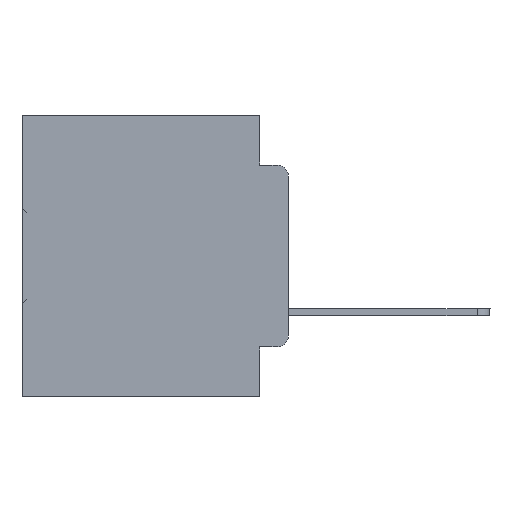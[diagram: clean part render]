
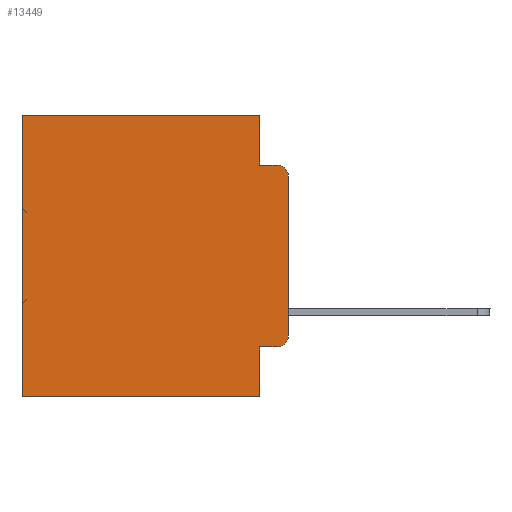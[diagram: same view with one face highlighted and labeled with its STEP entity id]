
A CAD part, left-side view. The second image highlights one B-rep face of the part: STEP entity #13449.
In plain terms, the highlighted planar face has unit normal (-1, 0, 0).
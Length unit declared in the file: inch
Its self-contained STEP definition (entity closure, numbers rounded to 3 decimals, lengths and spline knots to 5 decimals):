
#15 = CARTESIAN_POINT ( 'NONE',  ( 0.298, 0.051, -0.4115 ) ) ;
#1061 = ORIENTED_EDGE ( 'NONE', *, *, #3541, .F. ) ;
#1403 = FACE_OUTER_BOUND ( 'NONE', #36250, .T. ) ;
#1502 = CARTESIAN_POINT ( 'NONE',  ( 0.298, 0.051, -0.0885 ) ) ;
#1765 = AXIS2_PLACEMENT_3D ( 'NONE', #23868, #29611, #15576 ) ;
#1798 = LINE ( 'NONE', #21835, #19086 ) ;
#1844 = EDGE_CURVE ( 'NONE', #3510, #11392, #1798, .T. ) ;
#2751 = VECTOR ( 'NONE', #7389, 39.37008 ) ;
#3070 = CARTESIAN_POINT ( 'NONE',  ( 0.298, 0.473, -0.5 ) ) ;
#3287 = CARTESIAN_POINT ( 'NONE',  ( 0.298, 0., -0.1085 ) ) ;
#3510 = VERTEX_POINT ( 'NONE', #24153 ) ;
#3541 = EDGE_CURVE ( 'NONE', #10267, #5539, #7204, .T. ) ;
#3758 = CARTESIAN_POINT ( 'NONE',  ( 0.298, 0.02, -0.0885 ) ) ;
#4334 = VERTEX_POINT ( 'NONE', #31957 ) ;
#5153 = EDGE_CURVE ( 'NONE', #26758, #6152, #29954, .T. ) ;
#5460 = DIRECTION ( 'NONE',  ( -1., 0., 0. ) ) ;
#5539 = VERTEX_POINT ( 'NONE', #3070 ) ;
#5922 = EDGE_CURVE ( 'NONE', #33526, #5539, #17588, .T. ) ;
#6152 = VERTEX_POINT ( 'NONE', #3758 ) ;
#6642 = LINE ( 'NONE', #1502, #9301 ) ;
#7204 = LINE ( 'NONE', #13098, #2751 ) ;
#7389 = DIRECTION ( 'NONE',  ( 0., 1., 0. ) ) ;
#7728 = CARTESIAN_POINT ( 'NONE',  ( 0.298, 0.051, 0. ) ) ;
#8185 = DIRECTION ( 'NONE',  ( 0., 0., -1. ) ) ;
#8460 = EDGE_CURVE ( 'NONE', #3510, #33526, #17538, .T. ) ;
#8708 = VECTOR ( 'NONE', #18972, 39.37008 ) ;
#8750 = CARTESIAN_POINT ( 'NONE',  ( 0.298, 0.02, -0.3915 ) ) ;
#9301 = VECTOR ( 'NONE', #35219, 39.37008 ) ;
#9411 = CARTESIAN_POINT ( 'NONE',  ( 0.298, 0., 0. ) ) ;
#10267 = VERTEX_POINT ( 'NONE', #18409 ) ;
#10815 = DIRECTION ( 'NONE',  ( 0., 0., -1. ) ) ;
#11392 = VERTEX_POINT ( 'NONE', #24156 ) ;
#11633 = ORIENTED_EDGE ( 'NONE', *, *, #12539, .F. ) ;
#11670 = CARTESIAN_POINT ( 'NONE',  ( 0.298, 0.051, -0.4115 ) ) ;
#12088 = ORIENTED_EDGE ( 'NONE', *, *, #12703, .F. ) ;
#12374 = VECTOR ( 'NONE', #25185, 39.37008 ) ;
#12539 = EDGE_CURVE ( 'NONE', #11392, #6152, #6642, .T. ) ;
#12648 = PLANE ( 'NONE',  #1765 ) ;
#12703 = EDGE_CURVE ( 'NONE', #13671, #10267, #13623, .T. ) ;
#13098 = CARTESIAN_POINT ( 'NONE',  ( 0.298, 0., -0.5 ) ) ;
#13236 = CARTESIAN_POINT ( 'NONE',  ( 0.298, 0., 0. ) ) ;
#13449 = ADVANCED_FACE ( 'NONE', ( #1403 ), #12648, .F. ) ;
#13495 = ORIENTED_EDGE ( 'NONE', *, *, #1844, .F. ) ;
#13623 = LINE ( 'NONE', #7728, #8708 ) ;
#13671 = VERTEX_POINT ( 'NONE', #11670 ) ;
#14022 = ORIENTED_EDGE ( 'NONE', *, *, #8460, .T. ) ;
#14121 = ORIENTED_EDGE ( 'NONE', *, *, #5922, .T. ) ;
#14278 = ORIENTED_EDGE ( 'NONE', *, *, #5153, .T. ) ;
#14392 = EDGE_CURVE ( 'NONE', #26758, #17252, #27607, .T. ) ;
#14890 = CARTESIAN_POINT ( 'NONE',  ( 0.298, 0.02, -0.1085 ) ) ;
#15576 = DIRECTION ( 'NONE',  ( 0., 0., -1. ) ) ;
#16735 = ORIENTED_EDGE ( 'NONE', *, *, #14392, .F. ) ;
#16777 = LINE ( 'NONE', #15, #19523 ) ;
#16954 = DIRECTION ( 'NONE',  ( 0., -1., 0. ) ) ;
#17252 = VERTEX_POINT ( 'NONE', #24228 ) ;
#17538 = LINE ( 'NONE', #9411, #27428 ) ;
#17588 = LINE ( 'NONE', #20335, #26091 ) ;
#18409 = CARTESIAN_POINT ( 'NONE',  ( 0.298, 0.051, -0.5 ) ) ;
#18936 = EDGE_CURVE ( 'NONE', #4334, #17252, #34670, .T. ) ;
#18972 = DIRECTION ( 'NONE',  ( 0., 0., -1. ) ) ;
#19086 = VECTOR ( 'NONE', #8185, 39.37008 ) ;
#19523 = VECTOR ( 'NONE', #16954, 39.37008 ) ;
#20335 = CARTESIAN_POINT ( 'NONE',  ( 0.298, 0.473, 0. ) ) ;
#21713 = EDGE_CURVE ( 'NONE', #13671, #4334, #16777, .T. ) ;
#21835 = CARTESIAN_POINT ( 'NONE',  ( 0.298, 0.051, 0. ) ) ;
#22532 = DIRECTION ( 'NONE',  ( 0., 0., -1. ) ) ;
#23868 = CARTESIAN_POINT ( 'NONE',  ( 0.298, 0., 0. ) ) ;
#24037 = AXIS2_PLACEMENT_3D ( 'NONE', #14890, #26150, #31325 ) ;
#24153 = CARTESIAN_POINT ( 'NONE',  ( 0.298, 0.051, 0. ) ) ;
#24156 = CARTESIAN_POINT ( 'NONE',  ( 0.298, 0.051, -0.0885 ) ) ;
#24188 = ORIENTED_EDGE ( 'NONE', *, *, #21713, .T. ) ;
#24228 = CARTESIAN_POINT ( 'NONE',  ( 0.298, 0., -0.3915 ) ) ;
#24490 = ORIENTED_EDGE ( 'NONE', *, *, #18936, .T. ) ;
#25185 = DIRECTION ( 'NONE',  ( 0., 0., -1. ) ) ;
#26091 = VECTOR ( 'NONE', #22532, 39.37008 ) ;
#26150 = DIRECTION ( 'NONE',  ( -1., 0., 0. ) ) ;
#26758 = VERTEX_POINT ( 'NONE', #3287 ) ;
#27428 = VECTOR ( 'NONE', #28793, 39.37008 ) ;
#27607 = LINE ( 'NONE', #13236, #12374 ) ;
#28192 = AXIS2_PLACEMENT_3D ( 'NONE', #8750, #5460, #10815 ) ;
#28793 = DIRECTION ( 'NONE',  ( 0., 1., 0. ) ) ;
#29611 = DIRECTION ( 'NONE',  ( 1., 0., 0. ) ) ;
#29954 = CIRCLE ( 'NONE', #24037, 0.02 ) ;
#31325 = DIRECTION ( 'NONE',  ( 0., 0., -1. ) ) ;
#31957 = CARTESIAN_POINT ( 'NONE',  ( 0.298, 0.02, -0.4115 ) ) ;
#33525 = CARTESIAN_POINT ( 'NONE',  ( 0.298, 0.473, 0. ) ) ;
#33526 = VERTEX_POINT ( 'NONE', #33525 ) ;
#34670 = CIRCLE ( 'NONE', #28192, 0.02 ) ;
#35219 = DIRECTION ( 'NONE',  ( 0., -1., 0. ) ) ;
#36250 = EDGE_LOOP ( 'NONE', ( #16735, #14278, #11633, #13495, #14022, #14121, #1061, #12088, #24188, #24490 ) ) ;
